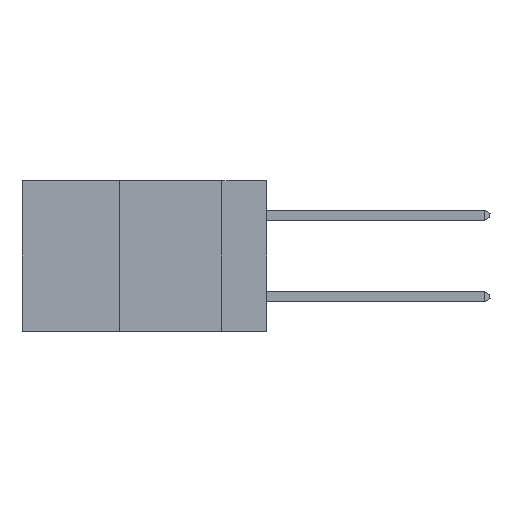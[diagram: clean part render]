
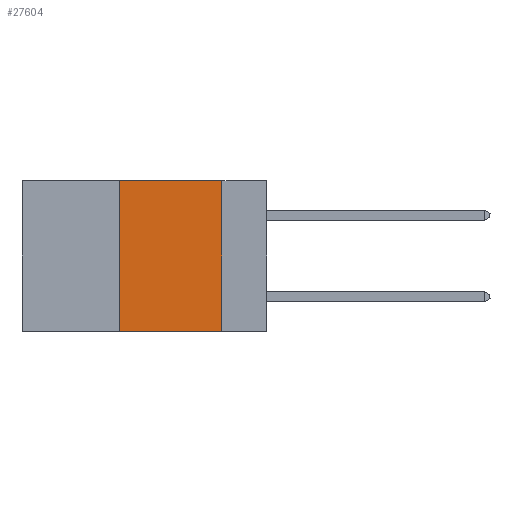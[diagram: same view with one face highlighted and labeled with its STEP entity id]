
A CAD part, left-side view. The second image highlights one B-rep face of the part: STEP entity #27604.
In plain terms, the highlighted planar face has unit normal (-1, 0, 0).
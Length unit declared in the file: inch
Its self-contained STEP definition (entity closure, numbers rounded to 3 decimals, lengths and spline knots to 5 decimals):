
#26 = ORIENTED_EDGE ( 'NONE', *, *, #21628, .F. ) ;
#1263 = DIRECTION ( 'NONE',  ( 1., 0., 0. ) ) ;
#5854 = FACE_OUTER_BOUND ( 'NONE', #16125, .T. ) ;
#10867 = LINE ( 'NONE', #21855, #40747 ) ;
#13070 = ORIENTED_EDGE ( 'NONE', *, *, #31131, .F. ) ;
#14276 = CARTESIAN_POINT ( 'NONE',  ( 0., 0.36, 0. ) ) ;
#14284 = DIRECTION ( 'NONE',  ( 0., -1., 0. ) ) ;
#16125 = EDGE_LOOP ( 'NONE', ( #13070, #25430, #26, #40047 ) ) ;
#16536 = VECTOR ( 'NONE', #18048, 39.37008 ) ;
#16702 = LINE ( 'NONE', #34898, #44189 ) ;
#18048 = DIRECTION ( 'NONE',  ( 0., 0., 1. ) ) ;
#18720 = EDGE_CURVE ( 'NONE', #33875, #38788, #10867, .T. ) ;
#19549 = CARTESIAN_POINT ( 'NONE',  ( 0., 0.36, -0.37 ) ) ;
#20100 = PLANE ( 'NONE',  #22168 ) ;
#21628 = EDGE_CURVE ( 'NONE', #33875, #36307, #26557, .T. ) ;
#21855 = CARTESIAN_POINT ( 'NONE',  ( 0., 0.6, -0.37 ) ) ;
#22168 = AXIS2_PLACEMENT_3D ( 'NONE', #46217, #1263, #27634 ) ;
#25430 = ORIENTED_EDGE ( 'NONE', *, *, #44686, .F. ) ;
#25450 = CARTESIAN_POINT ( 'NONE',  ( 0., 0.6, 0. ) ) ;
#26557 = LINE ( 'NONE', #14276, #16536 ) ;
#27604 = ADVANCED_FACE ( 'NONE', ( #5854 ), #20100, .F. ) ;
#27634 = DIRECTION ( 'NONE',  ( 0., 0., -1. ) ) ;
#29807 = CARTESIAN_POINT ( 'NONE',  ( 0., 0.11, -0.37 ) ) ;
#31131 = EDGE_CURVE ( 'NONE', #42741, #38788, #16702, .T. ) ;
#33875 = VERTEX_POINT ( 'NONE', #19549 ) ;
#34898 = CARTESIAN_POINT ( 'NONE',  ( 0., 0.11, 0. ) ) ;
#35876 = VECTOR ( 'NONE', #14284, 39.37008 ) ;
#36307 = VERTEX_POINT ( 'NONE', #41262 ) ;
#37233 = CARTESIAN_POINT ( 'NONE',  ( 0., 0.11, 0. ) ) ;
#38641 = DIRECTION ( 'NONE',  ( 0., 0., -1. ) ) ;
#38788 = VERTEX_POINT ( 'NONE', #29807 ) ;
#40047 = ORIENTED_EDGE ( 'NONE', *, *, #18720, .T. ) ;
#40747 = VECTOR ( 'NONE', #47965, 39.37008 ) ;
#41262 = CARTESIAN_POINT ( 'NONE',  ( 0., 0.36, 0. ) ) ;
#42741 = VERTEX_POINT ( 'NONE', #37233 ) ;
#44189 = VECTOR ( 'NONE', #38641, 39.37008 ) ;
#44686 = EDGE_CURVE ( 'NONE', #36307, #42741, #45781, .T. ) ;
#45781 = LINE ( 'NONE', #25450, #35876 ) ;
#46217 = CARTESIAN_POINT ( 'NONE',  ( 0., 0.6, 0. ) ) ;
#47965 = DIRECTION ( 'NONE',  ( 0., -1., 0. ) ) ;
